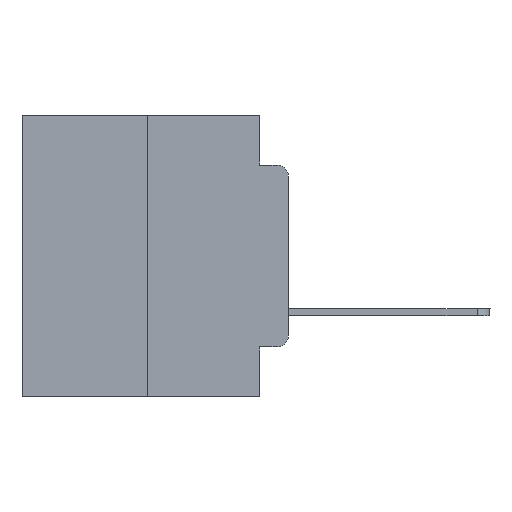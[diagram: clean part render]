
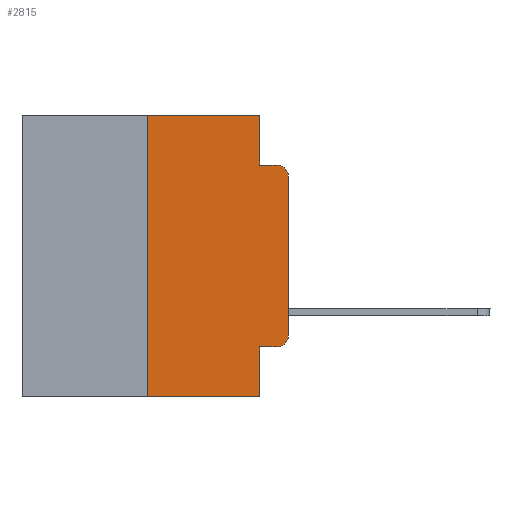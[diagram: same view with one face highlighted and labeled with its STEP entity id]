
A CAD part, left-side view. The second image highlights one B-rep face of the part: STEP entity #2815.
In plain terms, the highlighted planar face has unit normal (-1, 0, 0).
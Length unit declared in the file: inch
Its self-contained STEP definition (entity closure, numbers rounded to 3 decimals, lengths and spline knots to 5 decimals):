
#137 = VERTEX_POINT ( 'NONE', #2079 ) ;
#223 = VERTEX_POINT ( 'NONE', #21061 ) ;
#546 = CARTESIAN_POINT ( 'NONE',  ( 0., 0.051, -0.0885 ) ) ;
#897 = ORIENTED_EDGE ( 'NONE', *, *, #22369, .T. ) ;
#1025 = ORIENTED_EDGE ( 'NONE', *, *, #16115, .F. ) ;
#1205 = DIRECTION ( 'NONE',  ( -1., 0., 0. ) ) ;
#1376 = DIRECTION ( 'NONE',  ( 0., -1., 0. ) ) ;
#1410 = ORIENTED_EDGE ( 'NONE', *, *, #11863, .F. ) ;
#1522 = VECTOR ( 'NONE', #16393, 39.37008 ) ;
#1599 = VECTOR ( 'NONE', #25306, 39.37008 ) ;
#1955 = LINE ( 'NONE', #10517, #1522 ) ;
#2079 = CARTESIAN_POINT ( 'NONE',  ( 0., 0., -0.1085 ) ) ;
#2252 = EDGE_LOOP ( 'NONE', ( #897, #3499, #1410, #1025, #19220, #22857, #21913, #19462, #8797, #19999 ) ) ;
#2815 = ADVANCED_FACE ( 'NONE', ( #9234 ), #9622, .F. ) ;
#3350 = VERTEX_POINT ( 'NONE', #15351 ) ;
#3446 = CARTESIAN_POINT ( 'NONE',  ( 0., 0., 0. ) ) ;
#3499 = ORIENTED_EDGE ( 'NONE', *, *, #21983, .T. ) ;
#3892 = VERTEX_POINT ( 'NONE', #4695 ) ;
#4048 = LINE ( 'NONE', #17983, #25126 ) ;
#4205 = VECTOR ( 'NONE', #15802, 39.37008 ) ;
#4695 = CARTESIAN_POINT ( 'NONE',  ( 0., 0.25, -0.5 ) ) ;
#5037 = LINE ( 'NONE', #3446, #25600 ) ;
#5103 = LINE ( 'NONE', #23576, #1599 ) ;
#5734 = CARTESIAN_POINT ( 'NONE',  ( 0., 0.051, -0.5 ) ) ;
#5770 = EDGE_CURVE ( 'NONE', #3892, #3350, #1955, .T. ) ;
#5908 = AXIS2_PLACEMENT_3D ( 'NONE', #19788, #7482, #9383 ) ;
#6493 = VERTEX_POINT ( 'NONE', #21784 ) ;
#6792 = CIRCLE ( 'NONE', #7658, 0.02 ) ;
#7392 = DIRECTION ( 'NONE',  ( -1., 0., 0. ) ) ;
#7482 = DIRECTION ( 'NONE',  ( 1., 0., 0. ) ) ;
#7658 = AXIS2_PLACEMENT_3D ( 'NONE', #25712, #7392, #25184 ) ;
#7997 = LINE ( 'NONE', #11887, #17077 ) ;
#8797 = ORIENTED_EDGE ( 'NONE', *, *, #17418, .T. ) ;
#9234 = FACE_OUTER_BOUND ( 'NONE', #2252, .T. ) ;
#9358 = CARTESIAN_POINT ( 'NONE',  ( 0., 0.051, 0. ) ) ;
#9378 = VECTOR ( 'NONE', #25308, 39.37008 ) ;
#9383 = DIRECTION ( 'NONE',  ( 0., 0., -1. ) ) ;
#9622 = PLANE ( 'NONE',  #5908 ) ;
#10076 = EDGE_CURVE ( 'NONE', #3892, #13053, #5103, .T. ) ;
#10517 = CARTESIAN_POINT ( 'NONE',  ( 0., 0.25, 0. ) ) ;
#10656 = CARTESIAN_POINT ( 'NONE',  ( 0., 0., -0.3915 ) ) ;
#11096 = EDGE_CURVE ( 'NONE', #3350, #25471, #4048, .T. ) ;
#11480 = DIRECTION ( 'NONE',  ( 0., 0., 1. ) ) ;
#11863 = EDGE_CURVE ( 'NONE', #15033, #25774, #7997, .T. ) ;
#11887 = CARTESIAN_POINT ( 'NONE',  ( 0., 0.051, -0.0885 ) ) ;
#12356 = DIRECTION ( 'NONE',  ( 0., -1., 0. ) ) ;
#12802 = CARTESIAN_POINT ( 'NONE',  ( 0., 0.02, -0.0885 ) ) ;
#12953 = EDGE_CURVE ( 'NONE', #223, #15524, #22094, .T. ) ;
#13053 = VERTEX_POINT ( 'NONE', #5734 ) ;
#15033 = VERTEX_POINT ( 'NONE', #546 ) ;
#15351 = CARTESIAN_POINT ( 'NONE',  ( 0., 0.25, 0. ) ) ;
#15524 = VERTEX_POINT ( 'NONE', #10656 ) ;
#15541 = LINE ( 'NONE', #19701, #25647 ) ;
#15802 = DIRECTION ( 'NONE',  ( 0., 0., -1. ) ) ;
#16115 = EDGE_CURVE ( 'NONE', #25471, #15033, #17159, .T. ) ;
#16393 = DIRECTION ( 'NONE',  ( 0., 0., 1. ) ) ;
#17077 = VECTOR ( 'NONE', #22197, 39.37008 ) ;
#17159 = LINE ( 'NONE', #17682, #9378 ) ;
#17418 = EDGE_CURVE ( 'NONE', #6493, #223, #15541, .T. ) ;
#17682 = CARTESIAN_POINT ( 'NONE',  ( 0., 0.051, 0. ) ) ;
#17983 = CARTESIAN_POINT ( 'NONE',  ( 0., 0.473, 0. ) ) ;
#19220 = ORIENTED_EDGE ( 'NONE', *, *, #11096, .F. ) ;
#19462 = ORIENTED_EDGE ( 'NONE', *, *, #20204, .F. ) ;
#19701 = CARTESIAN_POINT ( 'NONE',  ( 0., 0.051, -0.4115 ) ) ;
#19788 = CARTESIAN_POINT ( 'NONE',  ( 0., 0.473, 0. ) ) ;
#19999 = ORIENTED_EDGE ( 'NONE', *, *, #12953, .T. ) ;
#20204 = EDGE_CURVE ( 'NONE', #6493, #13053, #25573, .T. ) ;
#21061 = CARTESIAN_POINT ( 'NONE',  ( 0., 0.02, -0.4115 ) ) ;
#21784 = CARTESIAN_POINT ( 'NONE',  ( 0., 0.051, -0.4115 ) ) ;
#21808 = CARTESIAN_POINT ( 'NONE',  ( 0., 0.02, -0.3915 ) ) ;
#21913 = ORIENTED_EDGE ( 'NONE', *, *, #10076, .T. ) ;
#21983 = EDGE_CURVE ( 'NONE', #137, #25774, #6792, .T. ) ;
#22094 = CIRCLE ( 'NONE', #26345, 0.02 ) ;
#22197 = DIRECTION ( 'NONE',  ( 0., -1., 0. ) ) ;
#22369 = EDGE_CURVE ( 'NONE', #15524, #137, #5037, .T. ) ;
#22857 = ORIENTED_EDGE ( 'NONE', *, *, #5770, .F. ) ;
#23576 = CARTESIAN_POINT ( 'NONE',  ( 0., 0.473, -0.5 ) ) ;
#23577 = CARTESIAN_POINT ( 'NONE',  ( 0., 0.051, 0. ) ) ;
#23944 = DIRECTION ( 'NONE',  ( 0., 0., -1. ) ) ;
#25126 = VECTOR ( 'NONE', #12356, 39.37008 ) ;
#25184 = DIRECTION ( 'NONE',  ( 0., 0., -1. ) ) ;
#25306 = DIRECTION ( 'NONE',  ( 0., -1., 0. ) ) ;
#25308 = DIRECTION ( 'NONE',  ( 0., 0., -1. ) ) ;
#25471 = VERTEX_POINT ( 'NONE', #9358 ) ;
#25573 = LINE ( 'NONE', #23577, #4205 ) ;
#25600 = VECTOR ( 'NONE', #11480, 39.37008 ) ;
#25647 = VECTOR ( 'NONE', #1376, 39.37008 ) ;
#25712 = CARTESIAN_POINT ( 'NONE',  ( 0., 0.02, -0.1085 ) ) ;
#25774 = VERTEX_POINT ( 'NONE', #12802 ) ;
#26345 = AXIS2_PLACEMENT_3D ( 'NONE', #21808, #1205, #23944 ) ;
